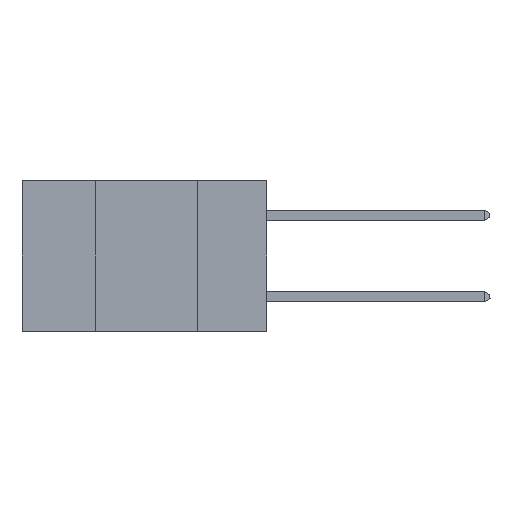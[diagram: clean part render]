
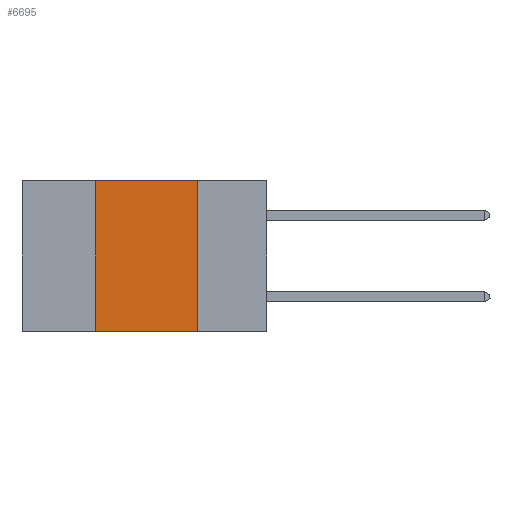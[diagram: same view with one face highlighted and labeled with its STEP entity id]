
A CAD part, left-side view. The second image highlights one B-rep face of the part: STEP entity #6695.
In plain terms, the highlighted planar face has unit normal (-1, 0, 0).
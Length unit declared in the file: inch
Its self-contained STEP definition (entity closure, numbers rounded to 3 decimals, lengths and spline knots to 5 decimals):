
#377 = DIRECTION ( 'NONE',  ( 0., 0., -1. ) ) ;
#480 = VERTEX_POINT ( 'NONE', #4498 ) ;
#2140 = CARTESIAN_POINT ( 'NONE',  ( 0., 0.6, 0. ) ) ;
#2474 = ORIENTED_EDGE ( 'NONE', *, *, #6141, .F. ) ;
#3602 = CARTESIAN_POINT ( 'NONE',  ( 0., 0.17, 0. ) ) ;
#4135 = ORIENTED_EDGE ( 'NONE', *, *, #15243, .F. ) ;
#4498 = CARTESIAN_POINT ( 'NONE',  ( 0., 0.42, 0. ) ) ;
#4892 = ORIENTED_EDGE ( 'NONE', *, *, #12261, .T. ) ;
#5214 = VERTEX_POINT ( 'NONE', #3602 ) ;
#5237 = PLANE ( 'NONE',  #11264 ) ;
#6110 = ORIENTED_EDGE ( 'NONE', *, *, #6701, .F. ) ;
#6141 = EDGE_CURVE ( 'NONE', #15143, #480, #7495, .T. ) ;
#6356 = CARTESIAN_POINT ( 'NONE',  ( 0., 0.17, 0. ) ) ;
#6695 = ADVANCED_FACE ( 'NONE', ( #15827 ), #5237, .F. ) ;
#6701 = EDGE_CURVE ( 'NONE', #5214, #6893, #12500, .T. ) ;
#6893 = VERTEX_POINT ( 'NONE', #13228 ) ;
#7123 = LINE ( 'NONE', #13041, #14134 ) ;
#7495 = LINE ( 'NONE', #15112, #8145 ) ;
#7733 = CARTESIAN_POINT ( 'NONE',  ( 0., 0.42, -0.37 ) ) ;
#7959 = VECTOR ( 'NONE', #12009, 39.37008 ) ;
#8145 = VECTOR ( 'NONE', #11119, 39.37008 ) ;
#8211 = LINE ( 'NONE', #2140, #7959 ) ;
#10158 = CARTESIAN_POINT ( 'NONE',  ( 0., 0.6, 0. ) ) ;
#11119 = DIRECTION ( 'NONE',  ( 0., 0., 1. ) ) ;
#11264 = AXIS2_PLACEMENT_3D ( 'NONE', #10158, #13965, #377 ) ;
#12009 = DIRECTION ( 'NONE',  ( 0., -1., 0. ) ) ;
#12261 = EDGE_CURVE ( 'NONE', #15143, #6893, #7123, .T. ) ;
#12500 = LINE ( 'NONE', #6356, #14895 ) ;
#12825 = DIRECTION ( 'NONE',  ( 0., 0., -1. ) ) ;
#13041 = CARTESIAN_POINT ( 'NONE',  ( 0., 0.6, -0.37 ) ) ;
#13119 = DIRECTION ( 'NONE',  ( 0., -1., 0. ) ) ;
#13228 = CARTESIAN_POINT ( 'NONE',  ( 0., 0.17, -0.37 ) ) ;
#13965 = DIRECTION ( 'NONE',  ( 1., 0., 0. ) ) ;
#14134 = VECTOR ( 'NONE', #13119, 39.37008 ) ;
#14895 = VECTOR ( 'NONE', #12825, 39.37008 ) ;
#15112 = CARTESIAN_POINT ( 'NONE',  ( 0., 0.42, 0. ) ) ;
#15143 = VERTEX_POINT ( 'NONE', #7733 ) ;
#15243 = EDGE_CURVE ( 'NONE', #480, #5214, #8211, .T. ) ;
#15680 = EDGE_LOOP ( 'NONE', ( #6110, #4135, #2474, #4892 ) ) ;
#15827 = FACE_OUTER_BOUND ( 'NONE', #15680, .T. ) ;
